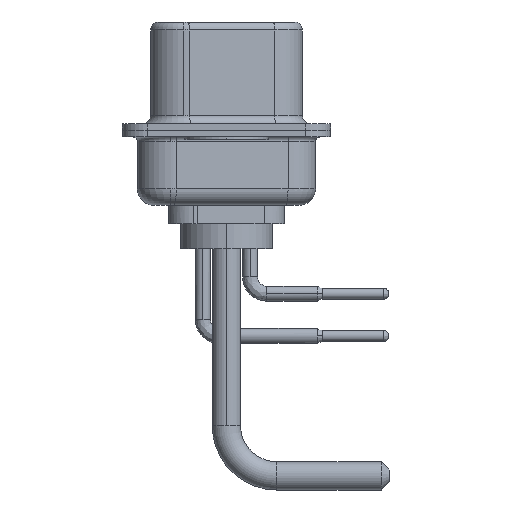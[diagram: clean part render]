
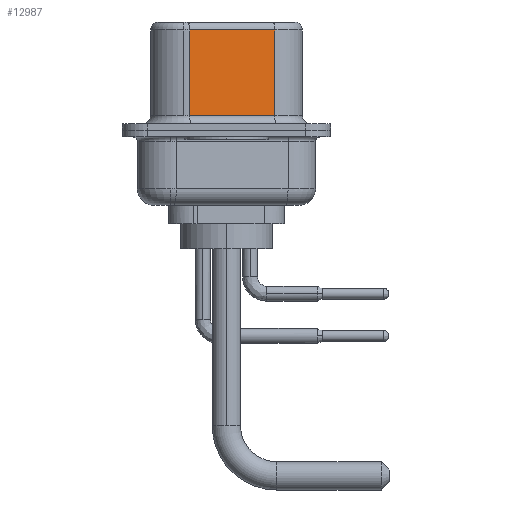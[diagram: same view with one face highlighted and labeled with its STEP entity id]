
A CAD part, left-side view. The second image highlights one B-rep face of the part: STEP entity #12987.
In plain terms, the highlighted planar face has unit normal (-0.985, -0.174, 0).
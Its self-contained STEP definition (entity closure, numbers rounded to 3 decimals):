
#1358 = EDGE_CURVE ( 'NONE', #14893, #6328, #4237, .T. ) ;
#1638 = CARTESIAN_POINT ( 'NONE',  ( 3.68, 2.203, 6.52 ) ) ;
#1771 = DIRECTION ( 'NONE',  ( 0.174, -0.985, 0. ) ) ;
#1832 = LINE ( 'NONE', #9533, #5575 ) ;
#2184 = ORIENTED_EDGE ( 'NONE', *, *, #13297, .T. ) ;
#3752 = VERTEX_POINT ( 'NONE', #18257 ) ;
#4237 = LINE ( 'NONE', #16100, #13912 ) ;
#4465 = DIRECTION ( 'NONE',  ( -0.174, 0.985, 0. ) ) ;
#4569 = CARTESIAN_POINT ( 'NONE',  ( 4.58, -2.897, 6.02 ) ) ;
#4716 = CARTESIAN_POINT ( 'NONE',  ( 4.58, -2.897, 6.52 ) ) ;
#5575 = VECTOR ( 'NONE', #17226, 1000. ) ;
#6240 = DIRECTION ( 'NONE',  ( -0.174, 0.985, 0. ) ) ;
#6328 = VERTEX_POINT ( 'NONE', #7813 ) ;
#7813 = CARTESIAN_POINT ( 'NONE',  ( 3.68, 2.203, 6.02 ) ) ;
#8313 = CARTESIAN_POINT ( 'NONE',  ( 4.58, -2.897, 0.9 ) ) ;
#8360 = EDGE_CURVE ( 'NONE', #6328, #3752, #15132, .T. ) ;
#9357 = ORIENTED_EDGE ( 'NONE', *, *, #17735, .F. ) ;
#9533 = CARTESIAN_POINT ( 'NONE',  ( 4.58, -2.897, 6.52 ) ) ;
#10060 = ORIENTED_EDGE ( 'NONE', *, *, #1358, .T. ) ;
#10812 = EDGE_LOOP ( 'NONE', ( #9357, #10060, #15664, #2184 ) ) ;
#11029 = VECTOR ( 'NONE', #11729, 1000. ) ;
#11729 = DIRECTION ( 'NONE',  ( 0., 0., -1. ) ) ;
#12285 = AXIS2_PLACEMENT_3D ( 'NONE', #4716, #21762, #4465 ) ;
#12987 = ADVANCED_FACE ( 'NONE', ( #16079 ), #23794, .F. ) ;
#13297 = EDGE_CURVE ( 'NONE', #3752, #22254, #18805, .T. ) ;
#13912 = VECTOR ( 'NONE', #6240, 1000. ) ;
#14893 = VERTEX_POINT ( 'NONE', #4569 ) ;
#15132 = LINE ( 'NONE', #1638, #11029 ) ;
#15664 = ORIENTED_EDGE ( 'NONE', *, *, #8360, .T. ) ;
#16079 = FACE_OUTER_BOUND ( 'NONE', #10812, .T. ) ;
#16100 = CARTESIAN_POINT ( 'NONE',  ( 4.58, -2.897, 6.02 ) ) ;
#16916 = CARTESIAN_POINT ( 'NONE',  ( 4.58, -2.897, 0.9 ) ) ;
#17226 = DIRECTION ( 'NONE',  ( 0., 0., -1. ) ) ;
#17735 = EDGE_CURVE ( 'NONE', #14893, #22254, #1832, .T. ) ;
#18257 = CARTESIAN_POINT ( 'NONE',  ( 3.68, 2.203, 0.9 ) ) ;
#18716 = VECTOR ( 'NONE', #1771, 1000. ) ;
#18805 = LINE ( 'NONE', #16916, #18716 ) ;
#21762 = DIRECTION ( 'NONE',  ( 0.985, 0.174, 0. ) ) ;
#22254 = VERTEX_POINT ( 'NONE', #8313 ) ;
#23794 = PLANE ( 'NONE',  #12285 ) ;
